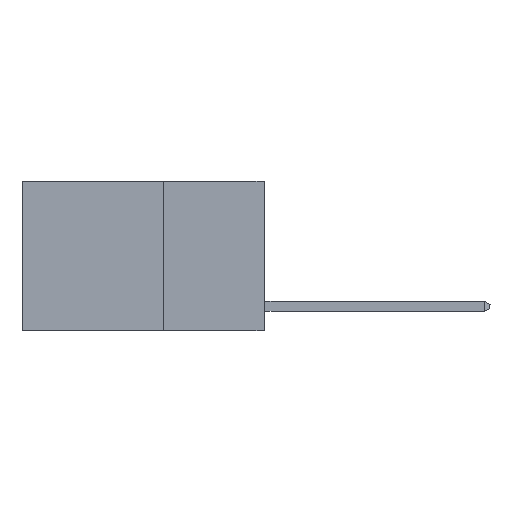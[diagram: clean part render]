
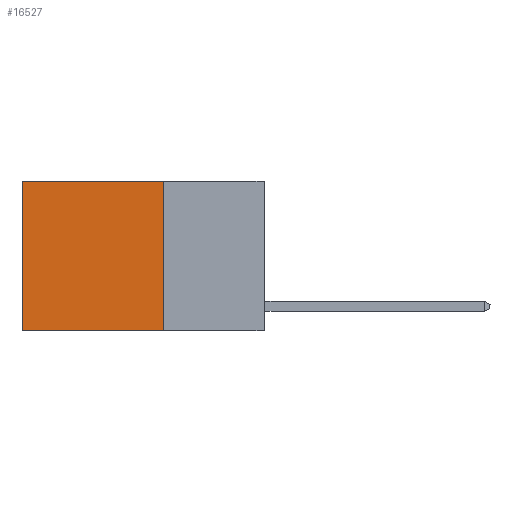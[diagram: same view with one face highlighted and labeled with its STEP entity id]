
A CAD part, left-side view. The second image highlights one B-rep face of the part: STEP entity #16527.
In plain terms, the highlighted planar face has unit normal (-1, 0, 0).
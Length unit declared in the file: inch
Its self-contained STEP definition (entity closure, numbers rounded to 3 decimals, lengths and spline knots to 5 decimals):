
#486 = CARTESIAN_POINT ( 'NONE',  ( 0.2625, 0.6, -0.37 ) ) ;
#2179 = EDGE_CURVE ( 'NONE', #8562, #6111, #8826, .T. ) ;
#2605 = CARTESIAN_POINT ( 'NONE',  ( 0.2625, 0.25, -0.37 ) ) ;
#2852 = EDGE_CURVE ( 'NONE', #17221, #11034, #9190, .T. ) ;
#3047 = DIRECTION ( 'NONE',  ( 0., 0., -1. ) ) ;
#3051 = FACE_OUTER_BOUND ( 'NONE', #8940, .T. ) ;
#5775 = EDGE_CURVE ( 'NONE', #17221, #8562, #14301, .T. ) ;
#5840 = LINE ( 'NONE', #7519, #13942 ) ;
#6111 = VERTEX_POINT ( 'NONE', #486 ) ;
#7400 = CARTESIAN_POINT ( 'NONE',  ( 0.2625, 0.25, 0. ) ) ;
#7468 = VECTOR ( 'NONE', #10530, 39.37008 ) ;
#7519 = CARTESIAN_POINT ( 'NONE',  ( 0.2625, 0.25, -0.37 ) ) ;
#7771 = CARTESIAN_POINT ( 'NONE',  ( 0.2625, 0.25, 0. ) ) ;
#8012 = DIRECTION ( 'NONE',  ( 1., 0., 0. ) ) ;
#8562 = VERTEX_POINT ( 'NONE', #14119 ) ;
#8694 = ORIENTED_EDGE ( 'NONE', *, *, #10055, .F. ) ;
#8826 = LINE ( 'NONE', #9721, #12847 ) ;
#8940 = EDGE_LOOP ( 'NONE', ( #13197, #8694, #13350, #12981 ) ) ;
#9190 = LINE ( 'NONE', #14091, #15800 ) ;
#9721 = CARTESIAN_POINT ( 'NONE',  ( 0.2625, 0.6, 0. ) ) ;
#10055 = EDGE_CURVE ( 'NONE', #11034, #6111, #5840, .T. ) ;
#10530 = DIRECTION ( 'NONE',  ( 0., 1., 0. ) ) ;
#11034 = VERTEX_POINT ( 'NONE', #2605 ) ;
#11467 = DIRECTION ( 'NONE',  ( 0., 0., -1. ) ) ;
#11600 = AXIS2_PLACEMENT_3D ( 'NONE', #16163, #8012, #13499 ) ;
#12231 = PLANE ( 'NONE',  #11600 ) ;
#12771 = DIRECTION ( 'NONE',  ( 0., 1., 0. ) ) ;
#12847 = VECTOR ( 'NONE', #3047, 39.37008 ) ;
#12981 = ORIENTED_EDGE ( 'NONE', *, *, #5775, .T. ) ;
#13197 = ORIENTED_EDGE ( 'NONE', *, *, #2179, .T. ) ;
#13350 = ORIENTED_EDGE ( 'NONE', *, *, #2852, .F. ) ;
#13499 = DIRECTION ( 'NONE',  ( 0., 0., -1. ) ) ;
#13942 = VECTOR ( 'NONE', #12771, 39.37008 ) ;
#14091 = CARTESIAN_POINT ( 'NONE',  ( 0.2625, 0.25, 0. ) ) ;
#14119 = CARTESIAN_POINT ( 'NONE',  ( 0.2625, 0.6, 0. ) ) ;
#14301 = LINE ( 'NONE', #7771, #7468 ) ;
#15800 = VECTOR ( 'NONE', #11467, 39.37008 ) ;
#16163 = CARTESIAN_POINT ( 'NONE',  ( 0.2625, 0.25, 0. ) ) ;
#16527 = ADVANCED_FACE ( 'NONE', ( #3051 ), #12231, .F. ) ;
#17221 = VERTEX_POINT ( 'NONE', #7400 ) ;
